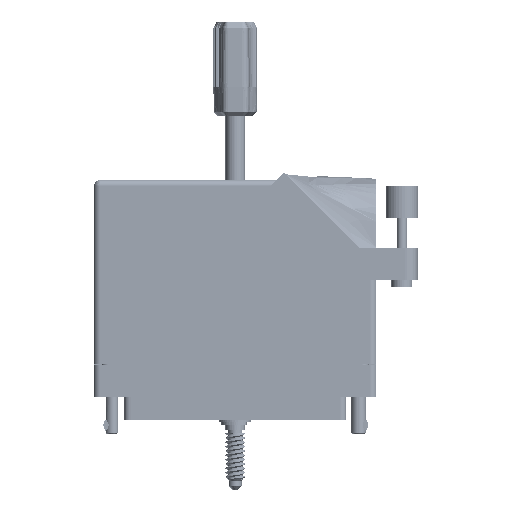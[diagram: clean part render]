
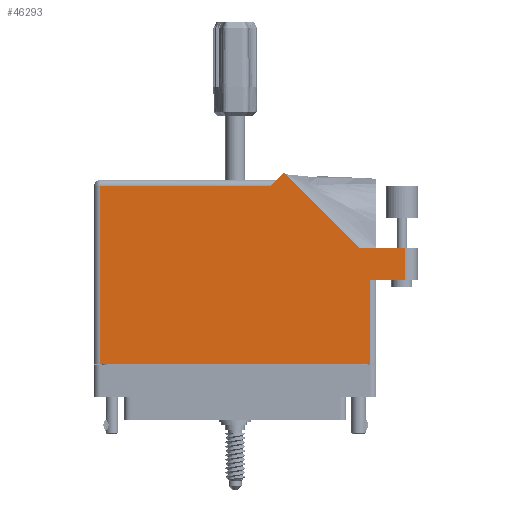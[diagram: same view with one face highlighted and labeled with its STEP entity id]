
A CAD part, front view. The second image highlights one B-rep face of the part: STEP entity #46293.
In plain terms, the highlighted face is planar.
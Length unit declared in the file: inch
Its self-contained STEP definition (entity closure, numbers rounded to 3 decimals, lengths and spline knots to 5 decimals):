
#1674 = ORIENTED_EDGE ( 'NONE', *, *, #7765, .T. ) ;
#2100 = VERTEX_POINT ( 'NONE', #24133 ) ;
#2942 = ORIENTED_EDGE ( 'NONE', *, *, #40522, .T. ) ;
#5267 = VECTOR ( 'NONE', #81874, 39.37008 ) ;
#6532 = ORIENTED_EDGE ( 'NONE', *, *, #24160, .T. ) ;
#7765 = EDGE_CURVE ( 'NONE', #64977, #77286, #72779, .T. ) ;
#8026 = CARTESIAN_POINT ( 'NONE',  ( 1.297, 0.715, 0.617 ) ) ;
#8632 = LINE ( 'NONE', #29739, #78783 ) ;
#9681 = CARTESIAN_POINT ( 'NONE',  ( -1.359, -0.1, 0.617 ) ) ;
#9703 = CARTESIAN_POINT ( 'NONE',  ( 1.19342, 1.022, 0.617 ) ) ;
#13620 = ORIENTED_EDGE ( 'NONE', *, *, #48285, .T. ) ;
#15096 = VECTOR ( 'NONE', #24424, 39.37008 ) ;
#15269 = LINE ( 'NONE', #39200, #52707 ) ;
#16491 = VECTOR ( 'NONE', #22791, 39.37008 ) ;
#19318 = DIRECTION ( 'NONE',  ( 0., -1., 0. ) ) ;
#19668 = CARTESIAN_POINT ( 'NONE',  ( -1.359, 1.675, 0.617 ) ) ;
#20872 = CARTESIAN_POINT ( 'NONE',  ( 1.759, 1.022, 0.617 ) ) ;
#21073 = CARTESIAN_POINT ( 'NONE',  ( 0.46971, 1.74571, 0.617 ) ) ;
#21424 = EDGE_CURVE ( 'NONE', #56629, #64977, #45803, .T. ) ;
#22791 = DIRECTION ( 'NONE',  ( 0., 1., 0. ) ) ;
#24133 = CARTESIAN_POINT ( 'NONE',  ( -1.297, -0.1, 0.617 ) ) ;
#24160 = EDGE_CURVE ( 'NONE', #52968, #39039, #40639, .T. ) ;
#24424 = DIRECTION ( 'NONE',  ( 1., 0., 0. ) ) ;
#25931 = DIRECTION ( 'NONE',  ( -1., 0., 0. ) ) ;
#26062 = CARTESIAN_POINT ( 'NONE',  ( -1.359, 1.613, 0.617 ) ) ;
#27865 = CARTESIAN_POINT ( 'NONE',  ( 0.337, 1.613, 0.617 ) ) ;
#27873 = CARTESIAN_POINT ( 'NONE',  ( -1.297, 1.613, 0.617 ) ) ;
#28256 = VECTOR ( 'NONE', #55470, 39.37008 ) ;
#28950 = EDGE_LOOP ( 'NONE', ( #1674, #36683, #6532, #13620, #87346, #79940, #81146, #2942, #33029 ) ) ;
#29739 = CARTESIAN_POINT ( 'NONE',  ( 1.19342, 1.022, 0.617 ) ) ;
#33029 = ORIENTED_EDGE ( 'NONE', *, *, #21424, .T. ) ;
#35033 = LINE ( 'NONE', #9681, #15096 ) ;
#36683 = ORIENTED_EDGE ( 'NONE', *, *, #47347, .T. ) ;
#39039 = VERTEX_POINT ( 'NONE', #9703 ) ;
#39200 = CARTESIAN_POINT ( 'NONE',  ( 0.399, 1.675, 0.617 ) ) ;
#40045 = AXIS2_PLACEMENT_3D ( 'NONE', #19668, #70651, #25931 ) ;
#40522 = EDGE_CURVE ( 'NONE', #2100, #56629, #35033, .T. ) ;
#40614 = PLANE ( 'NONE',  #40045 ) ;
#40639 = LINE ( 'NONE', #20872, #90893 ) ;
#44374 = LINE ( 'NONE', #65088, #91142 ) ;
#44649 = CARTESIAN_POINT ( 'NONE',  ( 1.297, 0.715, 0.617 ) ) ;
#45803 = LINE ( 'NONE', #8026, #16491 ) ;
#46293 = ADVANCED_FACE ( 'NONE', ( #54642 ), #40614, .F. ) ;
#47347 = EDGE_CURVE ( 'NONE', #77286, #52968, #62611, .T. ) ;
#48285 = EDGE_CURVE ( 'NONE', #39039, #90266, #8632, .T. ) ;
#50341 = CARTESIAN_POINT ( 'NONE',  ( 1.634, 1.022, 0.617 ) ) ;
#51234 = DIRECTION ( 'NONE',  ( -1., 0., 0. ) ) ;
#52707 = VECTOR ( 'NONE', #59754, 39.37008 ) ;
#52968 = VERTEX_POINT ( 'NONE', #50341 ) ;
#54642 = FACE_OUTER_BOUND ( 'NONE', #28950, .T. ) ;
#55470 = DIRECTION ( 'NONE',  ( -1., 0., 0. ) ) ;
#56629 = VERTEX_POINT ( 'NONE', #72041 ) ;
#56758 = CARTESIAN_POINT ( 'NONE',  ( 1.634, 0.715, 0.617 ) ) ;
#57301 = EDGE_CURVE ( 'NONE', #90266, #60091, #15269, .T. ) ;
#59754 = DIRECTION ( 'NONE',  ( -0.707, -0.707, 0. ) ) ;
#60091 = VERTEX_POINT ( 'NONE', #27865 ) ;
#62611 = LINE ( 'NONE', #81544, #5267 ) ;
#63348 = VERTEX_POINT ( 'NONE', #27873 ) ;
#63452 = VECTOR ( 'NONE', #92767, 39.37008 ) ;
#64977 = VERTEX_POINT ( 'NONE', #44649 ) ;
#65088 = CARTESIAN_POINT ( 'NONE',  ( -1.297, -0.1, 0.617 ) ) ;
#66847 = LINE ( 'NONE', #26062, #28256 ) ;
#67923 = EDGE_CURVE ( 'NONE', #63348, #2100, #44374, .T. ) ;
#70651 = DIRECTION ( 'NONE',  ( 0., 0., -1. ) ) ;
#72041 = CARTESIAN_POINT ( 'NONE',  ( 1.297, -0.1, 0.617 ) ) ;
#72779 = LINE ( 'NONE', #85213, #63452 ) ;
#75730 = DIRECTION ( 'NONE',  ( -0.707, 0.707, 0. ) ) ;
#77286 = VERTEX_POINT ( 'NONE', #56758 ) ;
#78783 = VECTOR ( 'NONE', #75730, 39.37008 ) ;
#79940 = ORIENTED_EDGE ( 'NONE', *, *, #80543, .T. ) ;
#80543 = EDGE_CURVE ( 'NONE', #60091, #63348, #66847, .T. ) ;
#81146 = ORIENTED_EDGE ( 'NONE', *, *, #67923, .T. ) ;
#81544 = CARTESIAN_POINT ( 'NONE',  ( 1.634, 1.022, 0.617 ) ) ;
#81874 = DIRECTION ( 'NONE',  ( 0., 1., 0. ) ) ;
#85213 = CARTESIAN_POINT ( 'NONE',  ( 1.359, 0.715, 0.617 ) ) ;
#87346 = ORIENTED_EDGE ( 'NONE', *, *, #57301, .T. ) ;
#90266 = VERTEX_POINT ( 'NONE', #21073 ) ;
#90893 = VECTOR ( 'NONE', #51234, 39.37008 ) ;
#91142 = VECTOR ( 'NONE', #19318, 39.37008 ) ;
#92767 = DIRECTION ( 'NONE',  ( 1., 0., 0. ) ) ;
